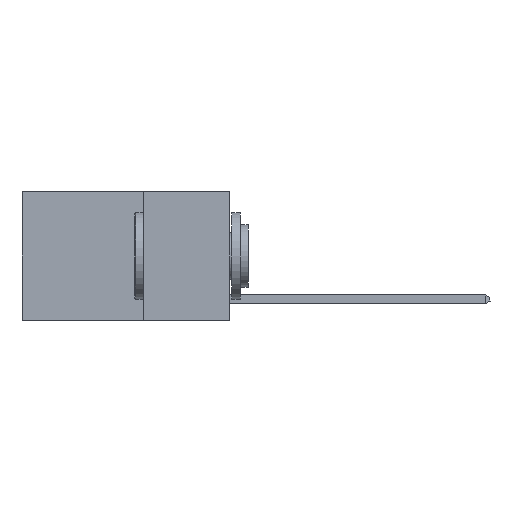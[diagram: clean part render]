
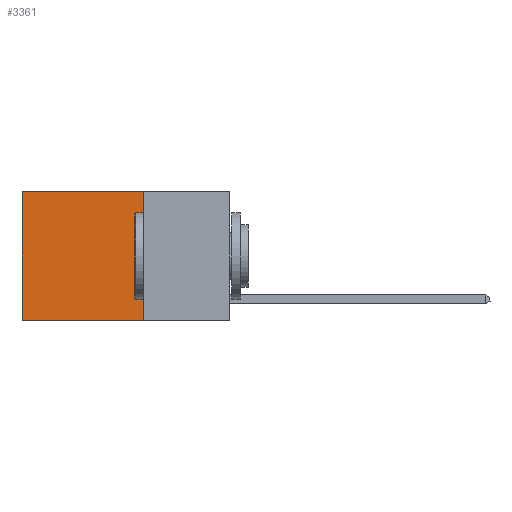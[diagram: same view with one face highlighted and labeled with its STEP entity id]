
A CAD part, left-side view. The second image highlights one B-rep face of the part: STEP entity #3361.
In plain terms, the highlighted planar face has unit normal (-1, 0, 0).
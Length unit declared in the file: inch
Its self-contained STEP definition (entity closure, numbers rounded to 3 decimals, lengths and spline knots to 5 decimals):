
#330 = CARTESIAN_POINT ( 'NONE',  ( 0.2625, 0.6, 0. ) ) ;
#920 = CARTESIAN_POINT ( 'NONE',  ( 0.2625, 0.25, 0. ) ) ;
#1471 = DIRECTION ( 'NONE',  ( 0., 0., -1. ) ) ;
#1858 = VECTOR ( 'NONE', #2317, 39.37008 ) ;
#2038 = ORIENTED_EDGE ( 'NONE', *, *, #6834, .T. ) ;
#2128 = ORIENTED_EDGE ( 'NONE', *, *, #2424, .F. ) ;
#2186 = ORIENTED_EDGE ( 'NONE', *, *, #9235, .F. ) ;
#2187 = ORIENTED_EDGE ( 'NONE', *, *, #11320, .T. ) ;
#2244 = VERTEX_POINT ( 'NONE', #5778 ) ;
#2317 = DIRECTION ( 'NONE',  ( 0., 1., 0. ) ) ;
#2424 = EDGE_CURVE ( 'NONE', #7643, #2244, #9903, .T. ) ;
#3361 = ADVANCED_FACE ( 'NONE', ( #9051 ), #9759, .F. ) ;
#3374 = CARTESIAN_POINT ( 'NONE',  ( 0.2625, 0.25, 0. ) ) ;
#3781 = EDGE_LOOP ( 'NONE', ( #2038, #2128, #2186, #2187 ) ) ;
#3998 = VERTEX_POINT ( 'NONE', #3374 ) ;
#4426 = CARTESIAN_POINT ( 'NONE',  ( 0.2625, 0.6, 0. ) ) ;
#4553 = LINE ( 'NONE', #330, #9264 ) ;
#5037 = VECTOR ( 'NONE', #11889, 39.37008 ) ;
#5348 = LINE ( 'NONE', #10969, #5037 ) ;
#5778 = CARTESIAN_POINT ( 'NONE',  ( 0.2625, 0.6, -0.37 ) ) ;
#5853 = CARTESIAN_POINT ( 'NONE',  ( 0.2625, 0.25, 0. ) ) ;
#6155 = DIRECTION ( 'NONE',  ( 1., 0., 0. ) ) ;
#6817 = AXIS2_PLACEMENT_3D ( 'NONE', #920, #6155, #12540 ) ;
#6829 = DIRECTION ( 'NONE',  ( 0., 1., 0. ) ) ;
#6834 = EDGE_CURVE ( 'NONE', #7464, #2244, #4553, .T. ) ;
#7464 = VERTEX_POINT ( 'NONE', #4426 ) ;
#7643 = VERTEX_POINT ( 'NONE', #8400 ) ;
#8400 = CARTESIAN_POINT ( 'NONE',  ( 0.2625, 0.25, -0.37 ) ) ;
#8839 = VECTOR ( 'NONE', #6829, 39.37008 ) ;
#9051 = FACE_OUTER_BOUND ( 'NONE', #3781, .T. ) ;
#9235 = EDGE_CURVE ( 'NONE', #3998, #7643, #5348, .T. ) ;
#9264 = VECTOR ( 'NONE', #1471, 39.37008 ) ;
#9759 = PLANE ( 'NONE',  #6817 ) ;
#9903 = LINE ( 'NONE', #11752, #1858 ) ;
#10969 = CARTESIAN_POINT ( 'NONE',  ( 0.2625, 0.25, 0. ) ) ;
#11202 = LINE ( 'NONE', #5853, #8839 ) ;
#11320 = EDGE_CURVE ( 'NONE', #3998, #7464, #11202, .T. ) ;
#11752 = CARTESIAN_POINT ( 'NONE',  ( 0.2625, 0.25, -0.37 ) ) ;
#11889 = DIRECTION ( 'NONE',  ( 0., 0., -1. ) ) ;
#12540 = DIRECTION ( 'NONE',  ( 0., 0., -1. ) ) ;
